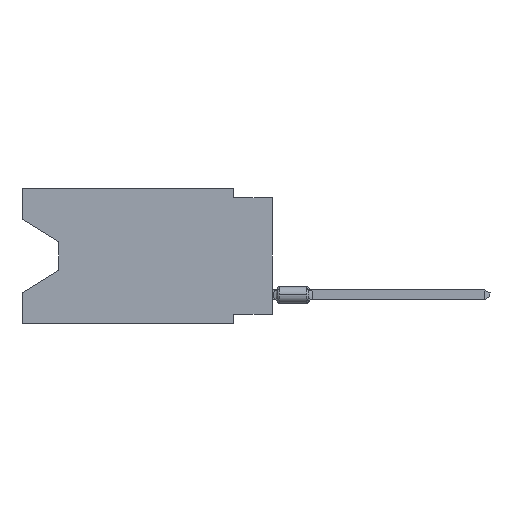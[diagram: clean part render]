
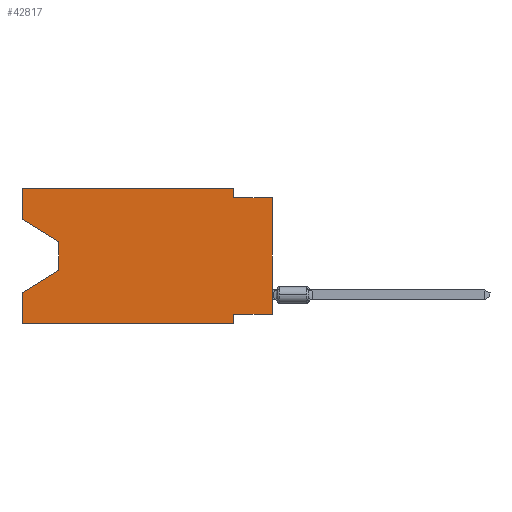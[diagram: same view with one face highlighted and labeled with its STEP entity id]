
A CAD part, left-side view. The second image highlights one B-rep face of the part: STEP entity #42817.
In plain terms, the highlighted planar face has unit normal (-1, 0, 0).
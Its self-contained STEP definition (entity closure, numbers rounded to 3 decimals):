
#2532 = VERTEX_POINT ( 'NONE', #10249 ) ;
#5646 = ORIENTED_EDGE ( 'NONE', *, *, #17515, .F. ) ;
#6265 = DIRECTION ( 'NONE',  ( 0., 0., -1. ) ) ;
#7792 = CARTESIAN_POINT ( 'NONE',  ( 0., 0., -0.635 ) ) ;
#9083 = CARTESIAN_POINT ( 'NONE',  ( 0., 13.97, -5.385 ) ) ;
#9871 = CARTESIAN_POINT ( 'NONE',  ( 0., 16.383, -8.89 ) ) ;
#10249 = CARTESIAN_POINT ( 'NONE',  ( 0., 13.97, -5.385 ) ) ;
#11956 = VECTOR ( 'NONE', #32146, 1000. ) ;
#12275 = CARTESIAN_POINT ( 'NONE',  ( 0., 13.97, -3.505 ) ) ;
#13736 = DIRECTION ( 'NONE',  ( 0., 0., 1. ) ) ;
#14180 = LINE ( 'NONE', #41343, #67487 ) ;
#14668 = VECTOR ( 'NONE', #22734, 1000. ) ;
#16942 = VERTEX_POINT ( 'NONE', #53661 ) ;
#16972 = ORIENTED_EDGE ( 'NONE', *, *, #19042, .F. ) ;
#17515 = EDGE_CURVE ( 'NONE', #77141, #36047, #67192, .T. ) ;
#19042 = EDGE_CURVE ( 'NONE', #58487, #37689, #42687, .T. ) ;
#19796 = ORIENTED_EDGE ( 'NONE', *, *, #107313, .F. ) ;
#20518 = VERTEX_POINT ( 'NONE', #95672 ) ;
#22582 = EDGE_CURVE ( 'NONE', #101098, #119148, #54979, .T. ) ;
#22734 = DIRECTION ( 'NONE',  ( 0., 0., 1. ) ) ;
#23114 = VECTOR ( 'NONE', #67154, 1000. ) ;
#28561 = DIRECTION ( 'NONE',  ( 1., 0., 0. ) ) ;
#30308 = CARTESIAN_POINT ( 'NONE',  ( 0., 16.383, -8.89 ) ) ;
#31720 = VECTOR ( 'NONE', #102032, 1000. ) ;
#31865 = CARTESIAN_POINT ( 'NONE',  ( 0., 2.54, 0. ) ) ;
#32146 = DIRECTION ( 'NONE',  ( 0., 0., 1. ) ) ;
#32267 = DIRECTION ( 'NONE',  ( 0., 0., -1. ) ) ;
#33690 = ORIENTED_EDGE ( 'NONE', *, *, #64417, .T. ) ;
#36047 = VERTEX_POINT ( 'NONE', #61062 ) ;
#37610 = PLANE ( 'NONE',  #63122 ) ;
#37689 = VERTEX_POINT ( 'NONE', #68191 ) ;
#38351 = CARTESIAN_POINT ( 'NONE',  ( 0., 2.54, -0.635 ) ) ;
#38419 = VERTEX_POINT ( 'NONE', #38351 ) ;
#41343 = CARTESIAN_POINT ( 'NONE',  ( 0., 2.54, -8.89 ) ) ;
#42029 = ORIENTED_EDGE ( 'NONE', *, *, #95195, .F. ) ;
#42687 = LINE ( 'NONE', #105443, #60166 ) ;
#42817 = ADVANCED_FACE ( 'NONE', ( #100989 ), #37610, .F. ) ;
#42864 = ORIENTED_EDGE ( 'NONE', *, *, #22582, .F. ) ;
#46496 = ORIENTED_EDGE ( 'NONE', *, *, #57664, .T. ) ;
#51426 = EDGE_CURVE ( 'NONE', #119148, #20518, #14180, .T. ) ;
#51435 = CARTESIAN_POINT ( 'NONE',  ( 0., 2.54, -8.255 ) ) ;
#51465 = DIRECTION ( 'NONE',  ( 0., -1., 0. ) ) ;
#53661 = CARTESIAN_POINT ( 'NONE',  ( 0., 2.54, 0. ) ) ;
#54979 = LINE ( 'NONE', #65213, #31720 ) ;
#55233 = CARTESIAN_POINT ( 'NONE',  ( 0., 16.383, -2.038 ) ) ;
#57664 = EDGE_CURVE ( 'NONE', #58487, #119024, #63007, .T. ) ;
#58487 = VERTEX_POINT ( 'NONE', #55233 ) ;
#58740 = CARTESIAN_POINT ( 'NONE',  ( 0., 16.383, 0. ) ) ;
#59635 = DIRECTION ( 'NONE',  ( 0., 0., -1. ) ) ;
#60166 = VECTOR ( 'NONE', #13736, 1000. ) ;
#60646 = CARTESIAN_POINT ( 'NONE',  ( 0., 16.383, -2.038 ) ) ;
#60683 = VECTOR ( 'NONE', #51465, 1000. ) ;
#61062 = CARTESIAN_POINT ( 'NONE',  ( 0., 16.383, -6.852 ) ) ;
#61086 = ORIENTED_EDGE ( 'NONE', *, *, #51426, .F. ) ;
#63007 = LINE ( 'NONE', #60646, #91399 ) ;
#63122 = AXIS2_PLACEMENT_3D ( 'NONE', #102790, #28561, #74418 ) ;
#64417 = EDGE_CURVE ( 'NONE', #2532, #36047, #99620, .T. ) ;
#65213 = CARTESIAN_POINT ( 'NONE',  ( 0., 0., -8.255 ) ) ;
#66913 = LINE ( 'NONE', #31865, #89437 ) ;
#67154 = DIRECTION ( 'NONE',  ( 0., -1., 0. ) ) ;
#67192 = LINE ( 'NONE', #58740, #11956 ) ;
#67487 = VECTOR ( 'NONE', #32267, 1000. ) ;
#68191 = CARTESIAN_POINT ( 'NONE',  ( 0., 16.383, 0. ) ) ;
#68416 = ORIENTED_EDGE ( 'NONE', *, *, #107679, .F. ) ;
#69170 = CARTESIAN_POINT ( 'NONE',  ( 0., 0., 0. ) ) ;
#69561 = CARTESIAN_POINT ( 'NONE',  ( 0., 16.383, 0. ) ) ;
#73157 = VERTEX_POINT ( 'NONE', #7792 ) ;
#74418 = DIRECTION ( 'NONE',  ( 0., 0., -1. ) ) ;
#76086 = EDGE_CURVE ( 'NONE', #101098, #73157, #96931, .T. ) ;
#77141 = VERTEX_POINT ( 'NONE', #30308 ) ;
#80474 = EDGE_LOOP ( 'NONE', ( #46496, #82210, #33690, #5646, #109844, #61086, #42864, #112082, #42029, #19796, #68416, #16972 ) ) ;
#80880 = EDGE_CURVE ( 'NONE', #77141, #20518, #111231, .T. ) ;
#82083 = DIRECTION ( 'NONE',  ( 0., 0.855, -0.519 ) ) ;
#82210 = ORIENTED_EDGE ( 'NONE', *, *, #102871, .T. ) ;
#86081 = CARTESIAN_POINT ( 'NONE',  ( 0., 0., -8.255 ) ) ;
#88923 = LINE ( 'NONE', #108230, #98372 ) ;
#89225 = CARTESIAN_POINT ( 'NONE',  ( 0., 0., -0.635 ) ) ;
#89437 = VECTOR ( 'NONE', #59635, 1000. ) ;
#89808 = DIRECTION ( 'NONE',  ( 0., -1., 0. ) ) ;
#91399 = VECTOR ( 'NONE', #98020, 1000. ) ;
#93408 = VECTOR ( 'NONE', #82083, 1000. ) ;
#95195 = EDGE_CURVE ( 'NONE', #38419, #73157, #115797, .T. ) ;
#95672 = CARTESIAN_POINT ( 'NONE',  ( 0., 2.54, -8.89 ) ) ;
#96931 = LINE ( 'NONE', #69170, #14668 ) ;
#98020 = DIRECTION ( 'NONE',  ( 0., -0.855, -0.519 ) ) ;
#98372 = VECTOR ( 'NONE', #6265, 1000. ) ;
#99620 = LINE ( 'NONE', #9083, #93408 ) ;
#100989 = FACE_OUTER_BOUND ( 'NONE', #80474, .T. ) ;
#101098 = VERTEX_POINT ( 'NONE', #86081 ) ;
#102032 = DIRECTION ( 'NONE',  ( 0., 1., 0. ) ) ;
#102790 = CARTESIAN_POINT ( 'NONE',  ( 0., 16.383, 0. ) ) ;
#102871 = EDGE_CURVE ( 'NONE', #119024, #2532, #88923, .T. ) ;
#105443 = CARTESIAN_POINT ( 'NONE',  ( 0., 16.383, 0. ) ) ;
#106377 = LINE ( 'NONE', #69561, #60683 ) ;
#107313 = EDGE_CURVE ( 'NONE', #16942, #38419, #66913, .T. ) ;
#107679 = EDGE_CURVE ( 'NONE', #37689, #16942, #106377, .T. ) ;
#108230 = CARTESIAN_POINT ( 'NONE',  ( 0., 13.97, -3.505 ) ) ;
#109844 = ORIENTED_EDGE ( 'NONE', *, *, #80880, .T. ) ;
#111231 = LINE ( 'NONE', #9871, #23114 ) ;
#112082 = ORIENTED_EDGE ( 'NONE', *, *, #76086, .T. ) ;
#115797 = LINE ( 'NONE', #89225, #118600 ) ;
#118600 = VECTOR ( 'NONE', #89808, 1000. ) ;
#119024 = VERTEX_POINT ( 'NONE', #12275 ) ;
#119148 = VERTEX_POINT ( 'NONE', #51435 ) ;
